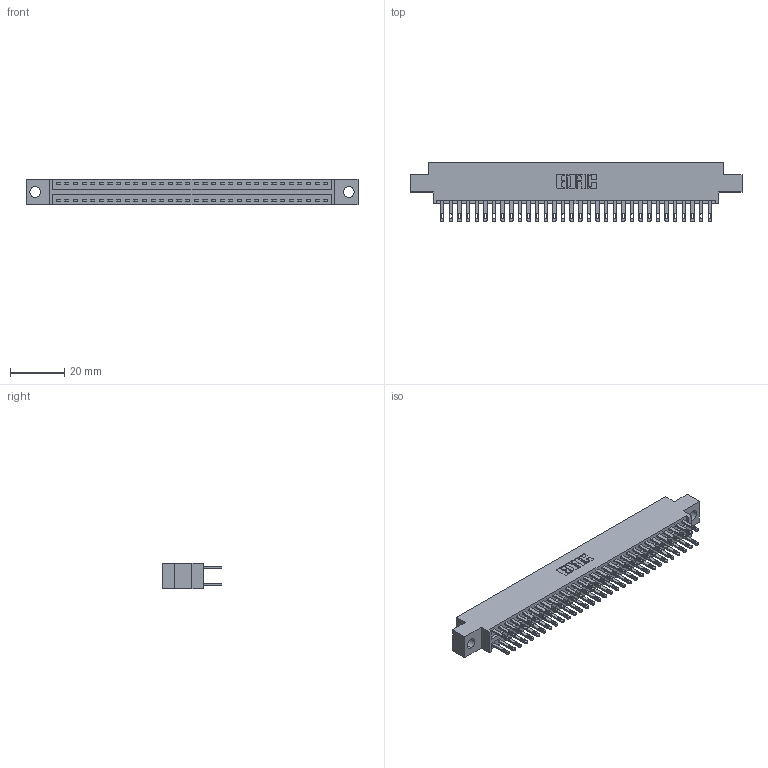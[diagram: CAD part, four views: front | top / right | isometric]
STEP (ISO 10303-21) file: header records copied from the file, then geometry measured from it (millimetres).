
FILE_DESCRIPTION (( 'STEP AP203' ), '1' );
FILE_NAME ('896-064-500-804.STEP', '2021-07-28T00:46:37', ( '' ), ( '' ), 'SwSTEP 2.0', 'SolidWorks 2020', '' );
FILE_SCHEMA (( 'CONFIG_CONTROL_DESIGN' ));
Length unit declared in the file: inch
Products named in the file (3): 846 Part_0.170 Offset - 0.156 Dia-TH; 345-292-001_345-293-100; 896-064-500-804
Assembly tree (65 placements, depth 2):
  896-064-500-804
    846 Part_0.170 Offset - 0.156 Dia-TH
    345-292-001_345-293-100  x64
Bounding box: 122.17 x 21.84 x 9.4 mm (x, y, z)
Volume: 11788.9 mm3; surface area: 16710.3 mm2
Topology: 65 solids, 65 shells, 3198 faces, 9749 edges, 6498 vertices
Faces by surface type: plane 1936, cylinder 1262
Entity records: 22295 total; most frequent: CARTESIAN_POINT 3688, ORIENTED_EDGE 3622, DIRECTION 3303, EDGE_CURVE 1811, VECTOR 1547, LINE 1547, VERTEX_POINT 1206, AXIS2_PLACEMENT_3D 878
